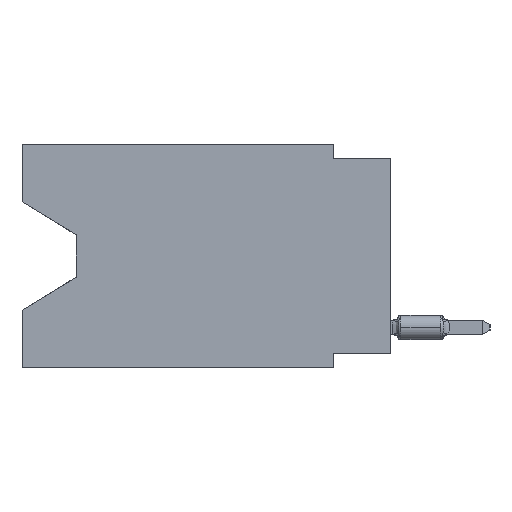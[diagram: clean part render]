
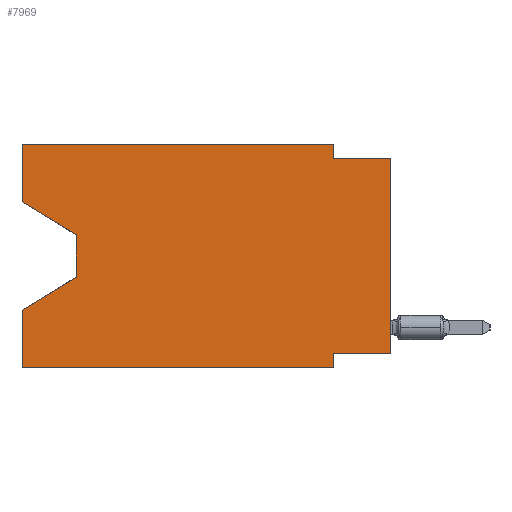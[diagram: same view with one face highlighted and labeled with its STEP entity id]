
A CAD part, left-side view. The second image highlights one B-rep face of the part: STEP entity #7969.
In plain terms, the highlighted planar face has unit normal (-1, 0, 0).
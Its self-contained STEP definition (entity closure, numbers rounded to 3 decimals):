
#960 = VECTOR ( 'NONE', #34333, 1000. ) ;
#1346 = DIRECTION ( 'NONE',  ( 0., -0.855, -0.519 ) ) ;
#2425 = ORIENTED_EDGE ( 'NONE', *, *, #37775, .T. ) ;
#2897 = CARTESIAN_POINT ( 'NONE',  ( 0., 16.383, 0. ) ) ;
#3836 = CARTESIAN_POINT ( 'NONE',  ( 0., 2.54, -9.271 ) ) ;
#4005 = DIRECTION ( 'NONE',  ( 0., 1., 0. ) ) ;
#4301 = ORIENTED_EDGE ( 'NONE', *, *, #16627, .F. ) ;
#4427 = VERTEX_POINT ( 'NONE', #29147 ) ;
#5253 = VERTEX_POINT ( 'NONE', #11702 ) ;
#5267 = ORIENTED_EDGE ( 'NONE', *, *, #31673, .T. ) ;
#5386 = VECTOR ( 'NONE', #17003, 1000. ) ;
#5451 = EDGE_CURVE ( 'NONE', #4427, #6808, #19205, .T. ) ;
#5868 = CARTESIAN_POINT ( 'NONE',  ( 0., 0., -0.635 ) ) ;
#5893 = VECTOR ( 'NONE', #9745, 1000. ) ;
#6417 = CARTESIAN_POINT ( 'NONE',  ( 0., 2.54, -9.906 ) ) ;
#6808 = VERTEX_POINT ( 'NONE', #7505 ) ;
#7505 = CARTESIAN_POINT ( 'NONE',  ( 0., 2.54, -0.635 ) ) ;
#7969 = ADVANCED_FACE ( 'NONE', ( #32698 ), #18204, .F. ) ;
#8187 = ORIENTED_EDGE ( 'NONE', *, *, #10342, .F. ) ;
#9745 = DIRECTION ( 'NONE',  ( 0., -1., 0. ) ) ;
#10342 = EDGE_CURVE ( 'NONE', #10373, #4427, #30593, .T. ) ;
#10373 = VERTEX_POINT ( 'NONE', #10378 ) ;
#10378 = CARTESIAN_POINT ( 'NONE',  ( 0., 16.383, 0. ) ) ;
#10398 = LINE ( 'NONE', #22386, #960 ) ;
#10850 = VERTEX_POINT ( 'NONE', #13470 ) ;
#11031 = DIRECTION ( 'NONE',  ( 0., 0.855, -0.519 ) ) ;
#11040 = ORIENTED_EDGE ( 'NONE', *, *, #18399, .F. ) ;
#11702 = CARTESIAN_POINT ( 'NONE',  ( 0., 16.383, -2.546 ) ) ;
#11808 = CARTESIAN_POINT ( 'NONE',  ( 0., 13.97, -4.013 ) ) ;
#12485 = ORIENTED_EDGE ( 'NONE', *, *, #18004, .F. ) ;
#13166 = EDGE_CURVE ( 'NONE', #10850, #28426, #16645, .T. ) ;
#13470 = CARTESIAN_POINT ( 'NONE',  ( 0., 16.383, -9.906 ) ) ;
#13501 = VECTOR ( 'NONE', #23077, 1000. ) ;
#13959 = CARTESIAN_POINT ( 'NONE',  ( 0., 13.97, -5.893 ) ) ;
#15566 = CARTESIAN_POINT ( 'NONE',  ( 0., 16.383, -7.36 ) ) ;
#15959 = VECTOR ( 'NONE', #28625, 1000. ) ;
#16513 = VERTEX_POINT ( 'NONE', #5868 ) ;
#16515 = VECTOR ( 'NONE', #29886, 1000. ) ;
#16627 = EDGE_CURVE ( 'NONE', #28681, #32092, #10398, .T. ) ;
#16645 = LINE ( 'NONE', #37225, #5386 ) ;
#16690 = EDGE_LOOP ( 'NONE', ( #18791, #2425, #5267, #37227, #22344, #4301, #11040, #33306, #19855, #37509, #8187, #12485 ) ) ;
#17003 = DIRECTION ( 'NONE',  ( 0., 0., 1. ) ) ;
#17814 = DIRECTION ( 'NONE',  ( 0., 0., -1. ) ) ;
#17938 = VECTOR ( 'NONE', #4005, 1000. ) ;
#18004 = EDGE_CURVE ( 'NONE', #5253, #10373, #19600, .T. ) ;
#18204 = PLANE ( 'NONE',  #27774 ) ;
#18242 = DIRECTION ( 'NONE',  ( 0., -1., 0. ) ) ;
#18399 = EDGE_CURVE ( 'NONE', #21434, #28681, #18960, .T. ) ;
#18791 = ORIENTED_EDGE ( 'NONE', *, *, #33160, .T. ) ;
#18960 = LINE ( 'NONE', #30913, #17938 ) ;
#18979 = VERTEX_POINT ( 'NONE', #35913 ) ;
#19029 = VECTOR ( 'NONE', #11031, 1000. ) ;
#19205 = LINE ( 'NONE', #37779, #29486 ) ;
#19600 = LINE ( 'NONE', #31552, #15959 ) ;
#19855 = ORIENTED_EDGE ( 'NONE', *, *, #25734, .F. ) ;
#20264 = LINE ( 'NONE', #13959, #19029 ) ;
#20597 = CARTESIAN_POINT ( 'NONE',  ( 0., 0., -9.271 ) ) ;
#21434 = VERTEX_POINT ( 'NONE', #20597 ) ;
#22344 = ORIENTED_EDGE ( 'NONE', *, *, #23992, .T. ) ;
#22386 = CARTESIAN_POINT ( 'NONE',  ( 0., 2.54, -9.906 ) ) ;
#22852 = VECTOR ( 'NONE', #1346, 1000. ) ;
#23077 = DIRECTION ( 'NONE',  ( 0., 0., 1. ) ) ;
#23468 = LINE ( 'NONE', #35213, #13501 ) ;
#23992 = EDGE_CURVE ( 'NONE', #10850, #32092, #24780, .T. ) ;
#24369 = DIRECTION ( 'NONE',  ( 0., -1., 0. ) ) ;
#24449 = CARTESIAN_POINT ( 'NONE',  ( 0., 16.383, 0. ) ) ;
#24780 = LINE ( 'NONE', #36529, #37192 ) ;
#25714 = LINE ( 'NONE', #31802, #22852 ) ;
#25734 = EDGE_CURVE ( 'NONE', #6808, #16513, #36637, .T. ) ;
#25996 = EDGE_CURVE ( 'NONE', #21434, #16513, #23468, .T. ) ;
#27774 = AXIS2_PLACEMENT_3D ( 'NONE', #24449, #30157, #17814 ) ;
#28426 = VERTEX_POINT ( 'NONE', #15566 ) ;
#28625 = DIRECTION ( 'NONE',  ( 0., 0., 1. ) ) ;
#28681 = VERTEX_POINT ( 'NONE', #3836 ) ;
#29147 = CARTESIAN_POINT ( 'NONE',  ( 0., 2.54, 0. ) ) ;
#29486 = VECTOR ( 'NONE', #31148, 1000. ) ;
#29886 = DIRECTION ( 'NONE',  ( 0., 0., -1. ) ) ;
#30157 = DIRECTION ( 'NONE',  ( 1., 0., 0. ) ) ;
#30593 = LINE ( 'NONE', #2897, #37722 ) ;
#30913 = CARTESIAN_POINT ( 'NONE',  ( 0., 0., -9.271 ) ) ;
#31148 = DIRECTION ( 'NONE',  ( 0., 0., -1. ) ) ;
#31552 = CARTESIAN_POINT ( 'NONE',  ( 0., 16.383, 0. ) ) ;
#31673 = EDGE_CURVE ( 'NONE', #18979, #28426, #20264, .T. ) ;
#31802 = CARTESIAN_POINT ( 'NONE',  ( 0., 16.383, -2.546 ) ) ;
#32092 = VERTEX_POINT ( 'NONE', #6417 ) ;
#32698 = FACE_OUTER_BOUND ( 'NONE', #16690, .T. ) ;
#33160 = EDGE_CURVE ( 'NONE', #5253, #36031, #25714, .T. ) ;
#33306 = ORIENTED_EDGE ( 'NONE', *, *, #25996, .T. ) ;
#34333 = DIRECTION ( 'NONE',  ( 0., 0., -1. ) ) ;
#35213 = CARTESIAN_POINT ( 'NONE',  ( 0., 0., 0. ) ) ;
#35787 = CARTESIAN_POINT ( 'NONE',  ( 0., 13.97, -4.013 ) ) ;
#35913 = CARTESIAN_POINT ( 'NONE',  ( 0., 13.97, -5.893 ) ) ;
#36031 = VERTEX_POINT ( 'NONE', #35787 ) ;
#36529 = CARTESIAN_POINT ( 'NONE',  ( 0., 16.383, -9.906 ) ) ;
#36637 = LINE ( 'NONE', #36839, #5893 ) ;
#36839 = CARTESIAN_POINT ( 'NONE',  ( 0., 0., -0.635 ) ) ;
#37192 = VECTOR ( 'NONE', #24369, 1000. ) ;
#37225 = CARTESIAN_POINT ( 'NONE',  ( 0., 16.383, 0. ) ) ;
#37227 = ORIENTED_EDGE ( 'NONE', *, *, #13166, .F. ) ;
#37509 = ORIENTED_EDGE ( 'NONE', *, *, #5451, .F. ) ;
#37722 = VECTOR ( 'NONE', #18242, 1000. ) ;
#37775 = EDGE_CURVE ( 'NONE', #36031, #18979, #38699, .T. ) ;
#37779 = CARTESIAN_POINT ( 'NONE',  ( 0., 2.54, 0. ) ) ;
#38699 = LINE ( 'NONE', #11808, #16515 ) ;
